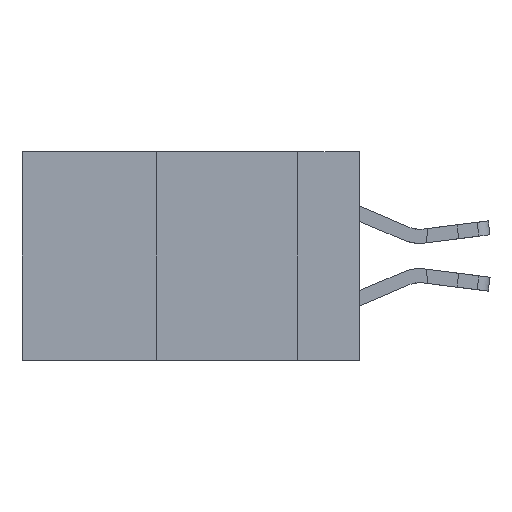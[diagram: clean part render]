
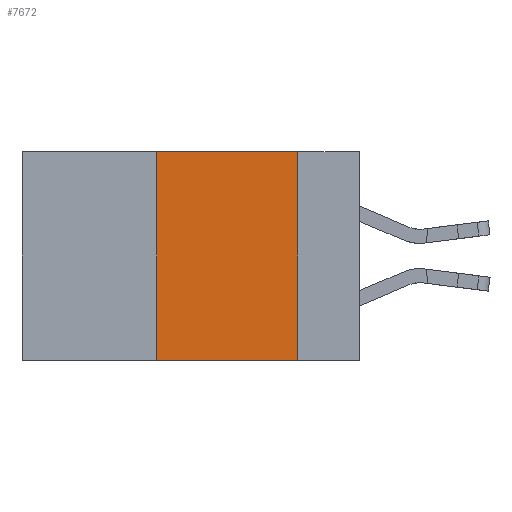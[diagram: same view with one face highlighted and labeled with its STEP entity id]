
A CAD part, left-side view. The second image highlights one B-rep face of the part: STEP entity #7672.
In plain terms, the highlighted planar face has unit normal (-1, 0, 0).
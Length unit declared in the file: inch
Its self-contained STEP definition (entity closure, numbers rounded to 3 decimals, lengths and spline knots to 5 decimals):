
#198 = VECTOR ( 'NONE', #20227, 39.37008 ) ;
#922 = AXIS2_PLACEMENT_3D ( 'NONE', #13233, #22480, #15751 ) ;
#1287 = CARTESIAN_POINT ( 'NONE',  ( 0., 0.6, 0. ) ) ;
#1446 = CARTESIAN_POINT ( 'NONE',  ( 0., 0.6, -0.37 ) ) ;
#1882 = CARTESIAN_POINT ( 'NONE',  ( 0., 0.36, -0.37 ) ) ;
#2224 = CARTESIAN_POINT ( 'NONE',  ( 0., 0.11, 0. ) ) ;
#2545 = ORIENTED_EDGE ( 'NONE', *, *, #2548, .T. ) ;
#2548 = EDGE_CURVE ( 'NONE', #18054, #4598, #6425, .T. ) ;
#4598 = VERTEX_POINT ( 'NONE', #10694 ) ;
#6070 = VERTEX_POINT ( 'NONE', #2224 ) ;
#6425 = LINE ( 'NONE', #1446, #198 ) ;
#7247 = VERTEX_POINT ( 'NONE', #11950 ) ;
#7672 = ADVANCED_FACE ( 'NONE', ( #15486 ), #22677, .F. ) ;
#8268 = CARTESIAN_POINT ( 'NONE',  ( 0., 0.11, 0. ) ) ;
#8331 = VECTOR ( 'NONE', #12481, 39.37008 ) ;
#8541 = LINE ( 'NONE', #8268, #29559 ) ;
#10694 = CARTESIAN_POINT ( 'NONE',  ( 0., 0.11, -0.37 ) ) ;
#11950 = CARTESIAN_POINT ( 'NONE',  ( 0., 0.36, 0. ) ) ;
#12214 = EDGE_CURVE ( 'NONE', #18054, #7247, #14458, .T. ) ;
#12310 = LINE ( 'NONE', #1287, #23192 ) ;
#12462 = EDGE_CURVE ( 'NONE', #7247, #6070, #12310, .T. ) ;
#12481 = DIRECTION ( 'NONE',  ( 0., 0., 1. ) ) ;
#13233 = CARTESIAN_POINT ( 'NONE',  ( 0., 0.6, 0. ) ) ;
#14458 = LINE ( 'NONE', #14676, #8331 ) ;
#14676 = CARTESIAN_POINT ( 'NONE',  ( 0., 0.36, 0. ) ) ;
#15486 = FACE_OUTER_BOUND ( 'NONE', #19028, .T. ) ;
#15751 = DIRECTION ( 'NONE',  ( 0., 0., -1. ) ) ;
#18054 = VERTEX_POINT ( 'NONE', #1882 ) ;
#19028 = EDGE_LOOP ( 'NONE', ( #23792, #22576, #26920, #2545 ) ) ;
#20227 = DIRECTION ( 'NONE',  ( 0., -1., 0. ) ) ;
#22480 = DIRECTION ( 'NONE',  ( 1., 0., 0. ) ) ;
#22576 = ORIENTED_EDGE ( 'NONE', *, *, #12462, .F. ) ;
#22677 = PLANE ( 'NONE',  #922 ) ;
#23192 = VECTOR ( 'NONE', #29700, 39.37008 ) ;
#23792 = ORIENTED_EDGE ( 'NONE', *, *, #29376, .F. ) ;
#26920 = ORIENTED_EDGE ( 'NONE', *, *, #12214, .F. ) ;
#29021 = DIRECTION ( 'NONE',  ( 0., 0., -1. ) ) ;
#29376 = EDGE_CURVE ( 'NONE', #6070, #4598, #8541, .T. ) ;
#29559 = VECTOR ( 'NONE', #29021, 39.37008 ) ;
#29700 = DIRECTION ( 'NONE',  ( 0., -1., 0. ) ) ;
